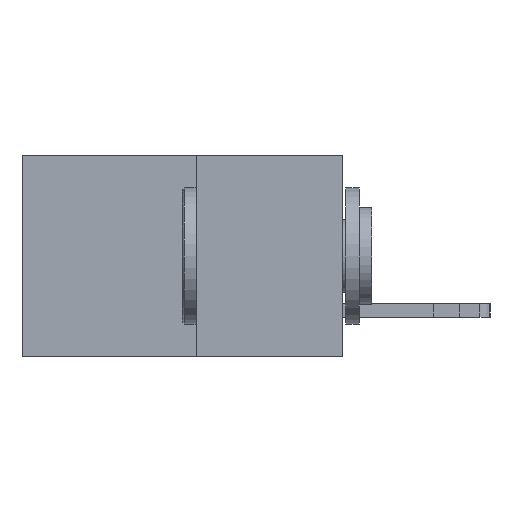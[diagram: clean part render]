
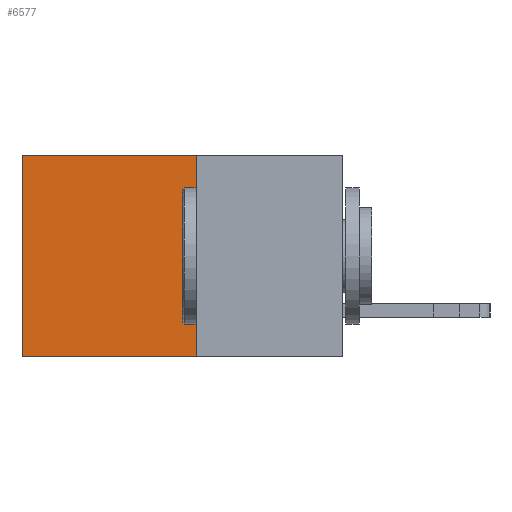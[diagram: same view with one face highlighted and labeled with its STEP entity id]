
A CAD part, left-side view. The second image highlights one B-rep face of the part: STEP entity #6577.
In plain terms, the highlighted planar face has unit normal (-1, 0, 0).
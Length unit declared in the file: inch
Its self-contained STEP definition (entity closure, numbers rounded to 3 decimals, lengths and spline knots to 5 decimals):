
#1076 = CARTESIAN_POINT ( 'NONE',  ( 0.277, 0.27, -0.37 ) ) ;
#1193 = VECTOR ( 'NONE', #10523, 39.37008 ) ;
#1481 = CARTESIAN_POINT ( 'NONE',  ( 0.277, 0.59, -0.37 ) ) ;
#2262 = AXIS2_PLACEMENT_3D ( 'NONE', #14429, #8114, #19242 ) ;
#2893 = EDGE_CURVE ( 'NONE', #12743, #13229, #14138, .T. ) ;
#3108 = CARTESIAN_POINT ( 'NONE',  ( 0.277, 0.59, -0.37 ) ) ;
#3937 = ORIENTED_EDGE ( 'NONE', *, *, #2893, .F. ) ;
#4281 = LINE ( 'NONE', #5477, #12427 ) ;
#4984 = LINE ( 'NONE', #1481, #8854 ) ;
#5282 = CARTESIAN_POINT ( 'NONE',  ( 0.277, 0.27, -0.37 ) ) ;
#5332 = FACE_OUTER_BOUND ( 'NONE', #9355, .T. ) ;
#5477 = CARTESIAN_POINT ( 'NONE',  ( 0.277, 0.27, -0.37 ) ) ;
#6577 = ADVANCED_FACE ( 'NONE', ( #5332 ), #17658, .F. ) ;
#7339 = ORIENTED_EDGE ( 'NONE', *, *, #7768, .F. ) ;
#7768 = EDGE_CURVE ( 'NONE', #19004, #12743, #4281, .T. ) ;
#8114 = DIRECTION ( 'NONE',  ( 1., 0., 0. ) ) ;
#8121 = VERTEX_POINT ( 'NONE', #12856 ) ;
#8751 = DIRECTION ( 'NONE',  ( 0., 1., 0. ) ) ;
#8854 = VECTOR ( 'NONE', #16057, 39.37008 ) ;
#9271 = ORIENTED_EDGE ( 'NONE', *, *, #14350, .T. ) ;
#9355 = EDGE_LOOP ( 'NONE', ( #13201, #3937, #7339, #9271 ) ) ;
#10523 = DIRECTION ( 'NONE',  ( 0., 1., 0. ) ) ;
#12427 = VECTOR ( 'NONE', #19888, 39.37008 ) ;
#12743 = VERTEX_POINT ( 'NONE', #5282 ) ;
#12856 = CARTESIAN_POINT ( 'NONE',  ( 0.277, 0.59, 0. ) ) ;
#13201 = ORIENTED_EDGE ( 'NONE', *, *, #15266, .T. ) ;
#13229 = VERTEX_POINT ( 'NONE', #3108 ) ;
#14138 = LINE ( 'NONE', #1076, #17826 ) ;
#14350 = EDGE_CURVE ( 'NONE', #19004, #8121, #17849, .T. ) ;
#14429 = CARTESIAN_POINT ( 'NONE',  ( 0.277, 0.27, -0.37 ) ) ;
#15266 = EDGE_CURVE ( 'NONE', #8121, #13229, #4984, .T. ) ;
#16057 = DIRECTION ( 'NONE',  ( 0., 0., -1. ) ) ;
#17658 = PLANE ( 'NONE',  #2262 ) ;
#17826 = VECTOR ( 'NONE', #8751, 39.37008 ) ;
#17849 = LINE ( 'NONE', #19978, #1193 ) ;
#18796 = CARTESIAN_POINT ( 'NONE',  ( 0.277, 0.27, 0. ) ) ;
#19004 = VERTEX_POINT ( 'NONE', #18796 ) ;
#19242 = DIRECTION ( 'NONE',  ( 0., 0., -1. ) ) ;
#19888 = DIRECTION ( 'NONE',  ( 0., 0., -1. ) ) ;
#19978 = CARTESIAN_POINT ( 'NONE',  ( 0.277, 0.27, 0. ) ) ;
